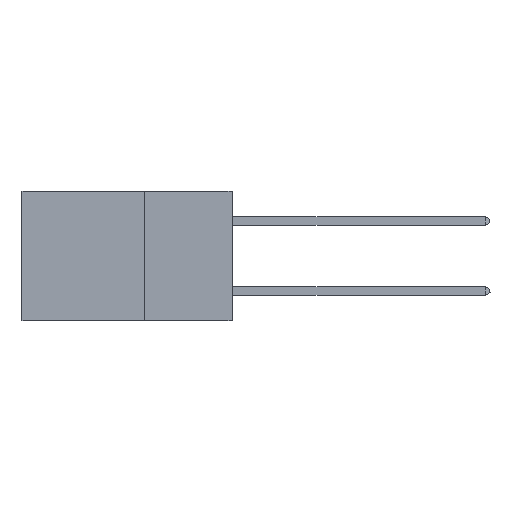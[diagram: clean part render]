
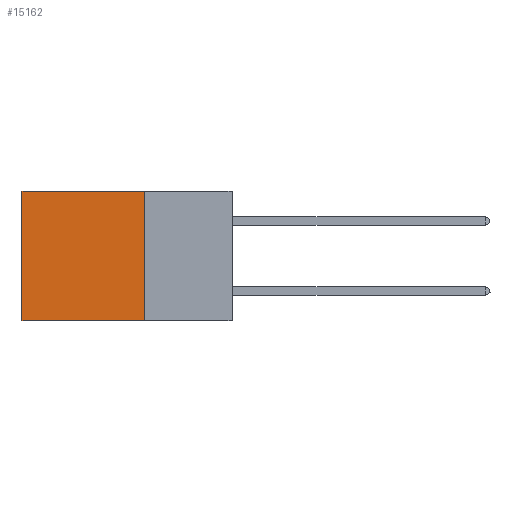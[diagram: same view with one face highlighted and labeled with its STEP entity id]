
A CAD part, left-side view. The second image highlights one B-rep face of the part: STEP entity #15162.
In plain terms, the highlighted planar face has unit normal (-1, 0, 0).
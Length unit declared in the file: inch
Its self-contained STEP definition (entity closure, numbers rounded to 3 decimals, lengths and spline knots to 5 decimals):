
#493 = DIRECTION ( 'NONE',  ( 0., 1., 0. ) ) ;
#656 = CARTESIAN_POINT ( 'NONE',  ( 0.2875, 0.6, 0. ) ) ;
#2045 = DIRECTION ( 'NONE',  ( 1., 0., 0. ) ) ;
#2197 = CARTESIAN_POINT ( 'NONE',  ( 0.2875, 0.25, 0. ) ) ;
#3042 = DIRECTION ( 'NONE',  ( 0., 0., -1. ) ) ;
#4119 = VERTEX_POINT ( 'NONE', #17398 ) ;
#4675 = LINE ( 'NONE', #16333, #7152 ) ;
#5136 = CARTESIAN_POINT ( 'NONE',  ( 0.2875, 0.25, -0.37 ) ) ;
#5266 = EDGE_LOOP ( 'NONE', ( #8855, #18750, #6832, #16759 ) ) ;
#5285 = DIRECTION ( 'NONE',  ( 0., 1., 0. ) ) ;
#5514 = LINE ( 'NONE', #17296, #16700 ) ;
#6832 = ORIENTED_EDGE ( 'NONE', *, *, #11999, .F. ) ;
#7080 = CARTESIAN_POINT ( 'NONE',  ( 0.2875, 0.6, 0. ) ) ;
#7152 = VECTOR ( 'NONE', #493, 39.37008 ) ;
#8387 = PLANE ( 'NONE',  #14348 ) ;
#8746 = VECTOR ( 'NONE', #5285, 39.37008 ) ;
#8855 = ORIENTED_EDGE ( 'NONE', *, *, #12028, .T. ) ;
#8957 = VECTOR ( 'NONE', #16726, 39.37008 ) ;
#9253 = LINE ( 'NONE', #2197, #8746 ) ;
#9864 = DIRECTION ( 'NONE',  ( 0., 0., -1. ) ) ;
#11999 = EDGE_CURVE ( 'NONE', #15751, #13610, #5514, .T. ) ;
#12028 = EDGE_CURVE ( 'NONE', #14714, #4119, #17140, .T. ) ;
#13610 = VERTEX_POINT ( 'NONE', #5136 ) ;
#14308 = CARTESIAN_POINT ( 'NONE',  ( 0.2875, 0.25, 0. ) ) ;
#14348 = AXIS2_PLACEMENT_3D ( 'NONE', #19464, #2045, #9864 ) ;
#14682 = EDGE_CURVE ( 'NONE', #15751, #14714, #9253, .T. ) ;
#14714 = VERTEX_POINT ( 'NONE', #7080 ) ;
#15162 = ADVANCED_FACE ( 'NONE', ( #15904 ), #8387, .F. ) ;
#15751 = VERTEX_POINT ( 'NONE', #14308 ) ;
#15904 = FACE_OUTER_BOUND ( 'NONE', #5266, .T. ) ;
#16333 = CARTESIAN_POINT ( 'NONE',  ( 0.2875, 0.25, -0.37 ) ) ;
#16700 = VECTOR ( 'NONE', #3042, 39.37008 ) ;
#16726 = DIRECTION ( 'NONE',  ( 0., 0., -1. ) ) ;
#16759 = ORIENTED_EDGE ( 'NONE', *, *, #14682, .T. ) ;
#17140 = LINE ( 'NONE', #656, #8957 ) ;
#17159 = EDGE_CURVE ( 'NONE', #13610, #4119, #4675, .T. ) ;
#17296 = CARTESIAN_POINT ( 'NONE',  ( 0.2875, 0.25, 0. ) ) ;
#17398 = CARTESIAN_POINT ( 'NONE',  ( 0.2875, 0.6, -0.37 ) ) ;
#18750 = ORIENTED_EDGE ( 'NONE', *, *, #17159, .F. ) ;
#19464 = CARTESIAN_POINT ( 'NONE',  ( 0.2875, 0.25, 0. ) ) ;
